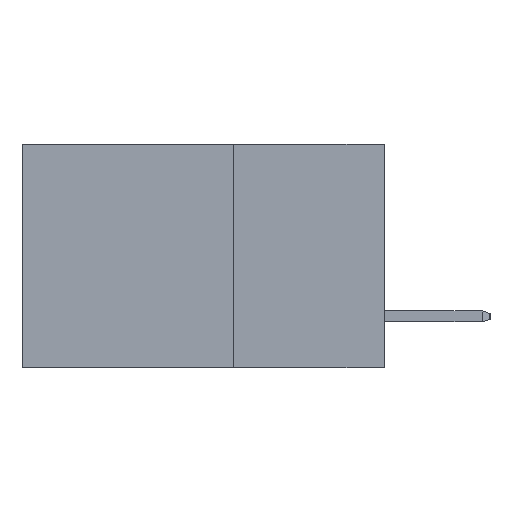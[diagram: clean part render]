
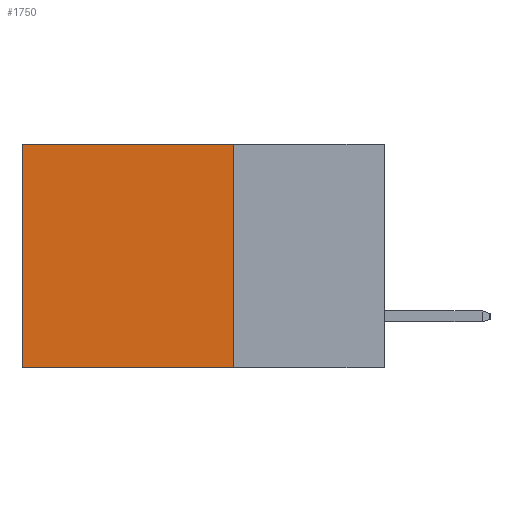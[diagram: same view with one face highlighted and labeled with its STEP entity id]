
A CAD part, left-side view. The second image highlights one B-rep face of the part: STEP entity #1750.
In plain terms, the highlighted planar face has unit normal (-1, 0, 0).
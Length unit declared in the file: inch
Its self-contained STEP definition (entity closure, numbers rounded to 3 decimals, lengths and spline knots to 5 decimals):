
#389 = LINE ( 'NONE', #12361, #6155 ) ;
#921 = ORIENTED_EDGE ( 'NONE', *, *, #11831, .F. ) ;
#1026 = DIRECTION ( 'NONE',  ( 0., 1., 0. ) ) ;
#1466 = DIRECTION ( 'NONE',  ( 0., 0., -1. ) ) ;
#1608 = CARTESIAN_POINT ( 'NONE',  ( 0.298, 0.25, 0. ) ) ;
#1670 = VERTEX_POINT ( 'NONE', #1704 ) ;
#1704 = CARTESIAN_POINT ( 'NONE',  ( 0.298, 0.25, 0. ) ) ;
#1728 = LINE ( 'NONE', #8495, #10061 ) ;
#1750 = ADVANCED_FACE ( 'NONE', ( #11775 ), #5648, .F. ) ;
#2128 = LINE ( 'NONE', #8619, #13669 ) ;
#2226 = VERTEX_POINT ( 'NONE', #9477 ) ;
#3220 = CARTESIAN_POINT ( 'NONE',  ( 0.298, 0.6, -0.37 ) ) ;
#3727 = AXIS2_PLACEMENT_3D ( 'NONE', #1608, #7760, #3798 ) ;
#3798 = DIRECTION ( 'NONE',  ( 0., 0., -1. ) ) ;
#4315 = CARTESIAN_POINT ( 'NONE',  ( 0.298, 0.25, -0.37 ) ) ;
#4676 = VERTEX_POINT ( 'NONE', #3220 ) ;
#4768 = ORIENTED_EDGE ( 'NONE', *, *, #8653, .T. ) ;
#5648 = PLANE ( 'NONE',  #3727 ) ;
#5751 = EDGE_LOOP ( 'NONE', ( #9940, #6309, #921, #4768 ) ) ;
#5776 = EDGE_CURVE ( 'NONE', #6368, #4676, #1728, .T. ) ;
#6007 = DIRECTION ( 'NONE',  ( 0., 0., -1. ) ) ;
#6155 = VECTOR ( 'NONE', #1466, 39.37008 ) ;
#6309 = ORIENTED_EDGE ( 'NONE', *, *, #8716, .F. ) ;
#6368 = VERTEX_POINT ( 'NONE', #13482 ) ;
#7760 = DIRECTION ( 'NONE',  ( 1., 0., 0. ) ) ;
#8495 = CARTESIAN_POINT ( 'NONE',  ( 0.298, 0.6, 0. ) ) ;
#8619 = CARTESIAN_POINT ( 'NONE',  ( 0.298, 0.25, 0. ) ) ;
#8653 = EDGE_CURVE ( 'NONE', #1670, #6368, #2128, .T. ) ;
#8716 = EDGE_CURVE ( 'NONE', #2226, #4676, #13001, .T. ) ;
#9477 = CARTESIAN_POINT ( 'NONE',  ( 0.298, 0.25, -0.37 ) ) ;
#9940 = ORIENTED_EDGE ( 'NONE', *, *, #5776, .T. ) ;
#10061 = VECTOR ( 'NONE', #6007, 39.37008 ) ;
#11775 = FACE_OUTER_BOUND ( 'NONE', #5751, .T. ) ;
#11831 = EDGE_CURVE ( 'NONE', #1670, #2226, #389, .T. ) ;
#12361 = CARTESIAN_POINT ( 'NONE',  ( 0.298, 0.25, 0. ) ) ;
#12671 = VECTOR ( 'NONE', #13039, 39.37008 ) ;
#13001 = LINE ( 'NONE', #4315, #12671 ) ;
#13039 = DIRECTION ( 'NONE',  ( 0., 1., 0. ) ) ;
#13482 = CARTESIAN_POINT ( 'NONE',  ( 0.298, 0.6, 0. ) ) ;
#13669 = VECTOR ( 'NONE', #1026, 39.37008 ) ;
